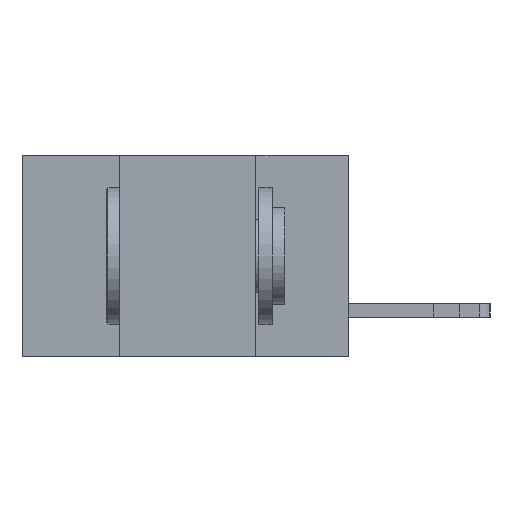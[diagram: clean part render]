
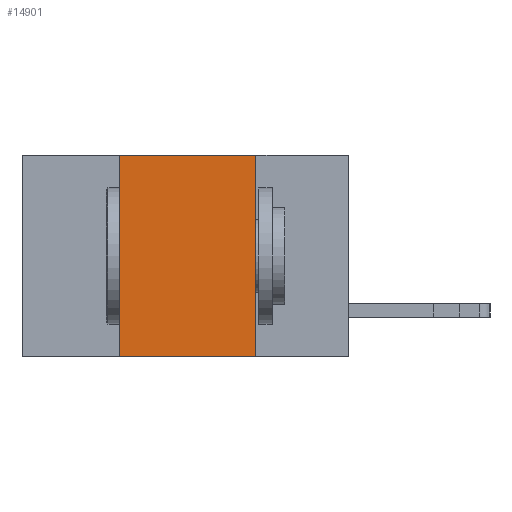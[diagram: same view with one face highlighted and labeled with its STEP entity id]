
A CAD part, left-side view. The second image highlights one B-rep face of the part: STEP entity #14901.
In plain terms, the highlighted planar face has unit normal (-1, 0, 0).
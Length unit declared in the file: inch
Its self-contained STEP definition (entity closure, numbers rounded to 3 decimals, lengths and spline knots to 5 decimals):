
#751 = AXIS2_PLACEMENT_3D ( 'NONE', #12387, #16510, #4463 ) ;
#1219 = EDGE_LOOP ( 'NONE', ( #23597, #17429, #11695, #21508 ) ) ;
#1488 = LINE ( 'NONE', #12673, #2752 ) ;
#1753 = LINE ( 'NONE', #2472, #22400 ) ;
#2043 = VERTEX_POINT ( 'NONE', #19469 ) ;
#2472 = CARTESIAN_POINT ( 'NONE',  ( 0., 0.6, 0. ) ) ;
#2752 = VECTOR ( 'NONE', #12440, 39.37008 ) ;
#3209 = EDGE_CURVE ( 'NONE', #6710, #3574, #5579, .T. ) ;
#3540 = EDGE_CURVE ( 'NONE', #2043, #3574, #1488, .T. ) ;
#3574 = VERTEX_POINT ( 'NONE', #4508 ) ;
#3705 = LINE ( 'NONE', #12651, #13718 ) ;
#4463 = DIRECTION ( 'NONE',  ( 0., 0., -1. ) ) ;
#4508 = CARTESIAN_POINT ( 'NONE',  ( 0., 0.17, -0.37 ) ) ;
#5579 = LINE ( 'NONE', #22939, #24924 ) ;
#6710 = VERTEX_POINT ( 'NONE', #21438 ) ;
#10380 = PLANE ( 'NONE',  #751 ) ;
#10545 = EDGE_CURVE ( 'NONE', #2043, #20714, #3705, .T. ) ;
#11695 = ORIENTED_EDGE ( 'NONE', *, *, #10545, .F. ) ;
#11711 = FACE_OUTER_BOUND ( 'NONE', #1219, .T. ) ;
#12387 = CARTESIAN_POINT ( 'NONE',  ( 0., 0.6, 0. ) ) ;
#12440 = DIRECTION ( 'NONE',  ( 0., -1., 0. ) ) ;
#12651 = CARTESIAN_POINT ( 'NONE',  ( 0., 0.42, 0. ) ) ;
#12673 = CARTESIAN_POINT ( 'NONE',  ( 0., 0.6, -0.37 ) ) ;
#13148 = DIRECTION ( 'NONE',  ( 0., 0., -1. ) ) ;
#13718 = VECTOR ( 'NONE', #20206, 39.37008 ) ;
#14901 = ADVANCED_FACE ( 'NONE', ( #11711 ), #10380, .F. ) ;
#14909 = EDGE_CURVE ( 'NONE', #20714, #6710, #1753, .T. ) ;
#15348 = CARTESIAN_POINT ( 'NONE',  ( 0., 0.42, 0. ) ) ;
#16510 = DIRECTION ( 'NONE',  ( 1., 0., 0. ) ) ;
#17429 = ORIENTED_EDGE ( 'NONE', *, *, #14909, .F. ) ;
#19469 = CARTESIAN_POINT ( 'NONE',  ( 0., 0.42, -0.37 ) ) ;
#20206 = DIRECTION ( 'NONE',  ( 0., 0., 1. ) ) ;
#20714 = VERTEX_POINT ( 'NONE', #15348 ) ;
#21438 = CARTESIAN_POINT ( 'NONE',  ( 0., 0.17, 0. ) ) ;
#21508 = ORIENTED_EDGE ( 'NONE', *, *, #3540, .T. ) ;
#22400 = VECTOR ( 'NONE', #24382, 39.37008 ) ;
#22939 = CARTESIAN_POINT ( 'NONE',  ( 0., 0.17, 0. ) ) ;
#23597 = ORIENTED_EDGE ( 'NONE', *, *, #3209, .F. ) ;
#24382 = DIRECTION ( 'NONE',  ( 0., -1., 0. ) ) ;
#24924 = VECTOR ( 'NONE', #13148, 39.37008 ) ;
